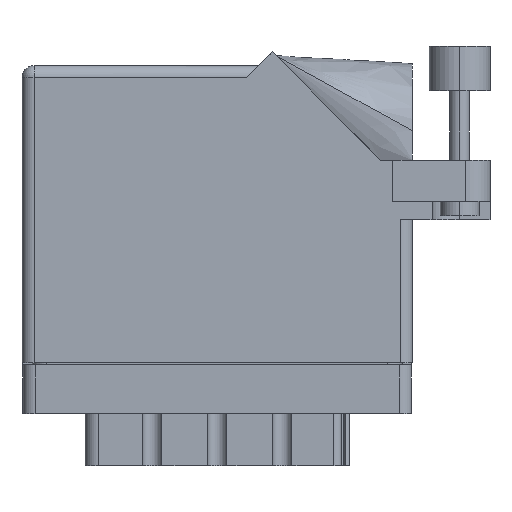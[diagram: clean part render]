
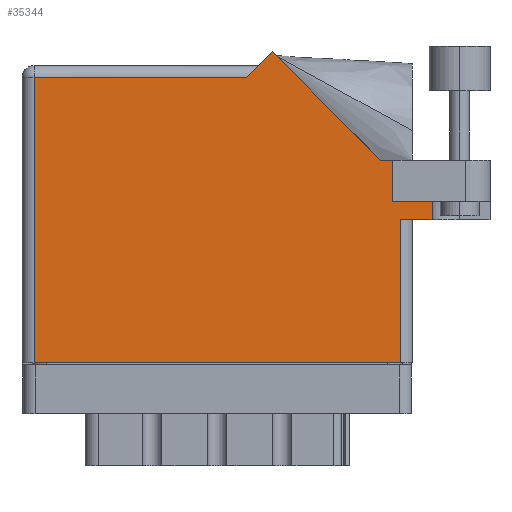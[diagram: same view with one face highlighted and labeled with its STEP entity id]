
A CAD part, front view. The second image highlights one B-rep face of the part: STEP entity #35344.
In plain terms, the highlighted face is planar.
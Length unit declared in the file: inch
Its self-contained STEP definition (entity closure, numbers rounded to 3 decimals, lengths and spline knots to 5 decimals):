
#977 = VERTEX_POINT ( 'NONE', #35370 ) ;
#1041 = CARTESIAN_POINT ( 'NONE',  ( 1.948, 0.737, 0. ) ) ;
#1799 = DIRECTION ( 'NONE',  ( 1., 0., 0. ) ) ;
#2195 = VECTOR ( 'NONE', #29705, 39.37008 ) ;
#2524 = CARTESIAN_POINT ( 'NONE',  ( 1.91, 0.831, 0. ) ) ;
#3030 = LINE ( 'NONE', #2524, #31104 ) ;
#3274 = VECTOR ( 'NONE', #40056, 39.37008 ) ;
#3302 = DIRECTION ( 'NONE',  ( 0., 0., -1. ) ) ;
#3703 = ORIENTED_EDGE ( 'NONE', *, *, #16335, .F. ) ;
#4080 = DIRECTION ( 'NONE',  ( -0.707, -0.707, 0. ) ) ;
#4946 = EDGE_CURVE ( 'NONE', #19174, #19849, #27779, .T. ) ;
#5634 = CARTESIAN_POINT ( 'NONE',  ( 1.84442, 1.044, 0. ) ) ;
#6701 = EDGE_CURVE ( 'NONE', #10170, #16494, #29284, .T. ) ;
#7838 = CARTESIAN_POINT ( 'NONE',  ( 2.01, 0.737, 0. ) ) ;
#8019 = VECTOR ( 'NONE', #28084, 39.37008 ) ;
#8037 = CARTESIAN_POINT ( 'NONE',  ( 1.84442, 1.044, 0. ) ) ;
#10122 = EDGE_CURVE ( 'NONE', #19849, #34673, #13090, .T. ) ;
#10170 = VERTEX_POINT ( 'NONE', #34140 ) ;
#11305 = DIRECTION ( 'NONE',  ( 0., -1., 0. ) ) ;
#11862 = CARTESIAN_POINT ( 'NONE',  ( 1.155, 1.468, 0. ) ) ;
#12029 = LINE ( 'NONE', #41518, #32100 ) ;
#12584 = LINE ( 'NONE', #23384, #13114 ) ;
#12904 = CARTESIAN_POINT ( 'NONE',  ( 1.28771, 1.60071, 0. ) ) ;
#13090 = LINE ( 'NONE', #5634, #8019 ) ;
#13114 = VECTOR ( 'NONE', #11305, 39.37008 ) ;
#13465 = EDGE_CURVE ( 'NONE', #977, #10170, #34619, .T. ) ;
#14250 = VERTEX_POINT ( 'NONE', #11862 ) ;
#14362 = VECTOR ( 'NONE', #4080, 39.37008 ) ;
#14633 = CARTESIAN_POINT ( 'NONE',  ( 1.948, 0., 0. ) ) ;
#15467 = ORIENTED_EDGE ( 'NONE', *, *, #37734, .T. ) ;
#15616 = VECTOR ( 'NONE', #40370, 39.37008 ) ;
#15752 = CARTESIAN_POINT ( 'NONE',  ( 2.1115, 0.831, 0. ) ) ;
#16335 = EDGE_CURVE ( 'NONE', #34590, #29541, #12029, .T. ) ;
#16494 = VERTEX_POINT ( 'NONE', #14633 ) ;
#17437 = EDGE_CURVE ( 'NONE', #32057, #32984, #25446, .T. ) ;
#17979 = CARTESIAN_POINT ( 'NONE',  ( 0., 1.468, 0. ) ) ;
#18394 = EDGE_CURVE ( 'NONE', #34673, #14250, #27894, .T. ) ;
#19174 = VERTEX_POINT ( 'NONE', #39757 ) ;
#19693 = CARTESIAN_POINT ( 'NONE',  ( 0., 1.53, 0. ) ) ;
#19698 = EDGE_LOOP ( 'NONE', ( #29198, #15467, #26949, #22063, #3703, #23926, #40928, #27675, #39932, #21300, #20784 ) ) ;
#19849 = VERTEX_POINT ( 'NONE', #8037 ) ;
#19925 = VECTOR ( 'NONE', #1799, 39.37008 ) ;
#20784 = ORIENTED_EDGE ( 'NONE', *, *, #13465, .T. ) ;
#20928 = DIRECTION ( 'NONE',  ( 1., 0., 0. ) ) ;
#21300 = ORIENTED_EDGE ( 'NONE', *, *, #29539, .T. ) ;
#22063 = ORIENTED_EDGE ( 'NONE', *, *, #23149, .F. ) ;
#22115 = CARTESIAN_POINT ( 'NONE',  ( 1.91, 0.831, 0. ) ) ;
#22775 = VECTOR ( 'NONE', #20928, 39.37008 ) ;
#23149 = EDGE_CURVE ( 'NONE', #29541, #32984, #12584, .T. ) ;
#23384 = CARTESIAN_POINT ( 'NONE',  ( 2.1115, 1.16177, 0. ) ) ;
#23541 = EDGE_CURVE ( 'NONE', #34590, #19174, #3030, .T. ) ;
#23926 = ORIENTED_EDGE ( 'NONE', *, *, #23541, .T. ) ;
#24104 = LINE ( 'NONE', #17979, #15616 ) ;
#25446 = LINE ( 'NONE', #7838, #19925 ) ;
#26949 = ORIENTED_EDGE ( 'NONE', *, *, #17437, .T. ) ;
#27675 = ORIENTED_EDGE ( 'NONE', *, *, #10122, .T. ) ;
#27779 = LINE ( 'NONE', #39233, #2195 ) ;
#27894 = LINE ( 'NONE', #39392, #14362 ) ;
#28084 = DIRECTION ( 'NONE',  ( -0.707, 0.707, 0. ) ) ;
#28973 = AXIS2_PLACEMENT_3D ( 'NONE', #19693, #3302, #32335 ) ;
#29198 = ORIENTED_EDGE ( 'NONE', *, *, #6701, .T. ) ;
#29284 = LINE ( 'NONE', #40127, #22775 ) ;
#29539 = EDGE_CURVE ( 'NONE', #14250, #977, #24104, .T. ) ;
#29541 = VERTEX_POINT ( 'NONE', #15752 ) ;
#29705 = DIRECTION ( 'NONE',  ( -1., 0., 0. ) ) ;
#30269 = CARTESIAN_POINT ( 'NONE',  ( 1.948, 0.737, 0. ) ) ;
#31104 = VECTOR ( 'NONE', #38386, 39.37008 ) ;
#31481 = CARTESIAN_POINT ( 'NONE',  ( 0.062, 0., 0. ) ) ;
#32057 = VERTEX_POINT ( 'NONE', #1041 ) ;
#32100 = VECTOR ( 'NONE', #38863, 39.37008 ) ;
#32335 = DIRECTION ( 'NONE',  ( -1., 0., 0. ) ) ;
#32984 = VERTEX_POINT ( 'NONE', #35993 ) ;
#34119 = VECTOR ( 'NONE', #38738, 39.37008 ) ;
#34140 = CARTESIAN_POINT ( 'NONE',  ( 0.062, 0., 0. ) ) ;
#34590 = VERTEX_POINT ( 'NONE', #22115 ) ;
#34619 = LINE ( 'NONE', #31481, #34119 ) ;
#34673 = VERTEX_POINT ( 'NONE', #12904 ) ;
#35344 = ADVANCED_FACE ( 'NONE', ( #36517 ), #35405, .F. ) ;
#35370 = CARTESIAN_POINT ( 'NONE',  ( 0.062, 1.468, 0. ) ) ;
#35405 = PLANE ( 'NONE',  #28973 ) ;
#35993 = CARTESIAN_POINT ( 'NONE',  ( 2.1115, 0.737, 0. ) ) ;
#36517 = FACE_OUTER_BOUND ( 'NONE', #19698, .T. ) ;
#37368 = LINE ( 'NONE', #30269, #3274 ) ;
#37734 = EDGE_CURVE ( 'NONE', #16494, #32057, #37368, .T. ) ;
#38386 = DIRECTION ( 'NONE',  ( 0., 1., 0. ) ) ;
#38738 = DIRECTION ( 'NONE',  ( 0., -1., 0. ) ) ;
#38863 = DIRECTION ( 'NONE',  ( 1., 0., 0. ) ) ;
#39233 = CARTESIAN_POINT ( 'NONE',  ( 2.41, 1.044, 0. ) ) ;
#39392 = CARTESIAN_POINT ( 'NONE',  ( 1.217, 1.53, 0. ) ) ;
#39757 = CARTESIAN_POINT ( 'NONE',  ( 1.91, 1.044, 0. ) ) ;
#39932 = ORIENTED_EDGE ( 'NONE', *, *, #18394, .T. ) ;
#40056 = DIRECTION ( 'NONE',  ( 0., 1., 0. ) ) ;
#40127 = CARTESIAN_POINT ( 'NONE',  ( 0., 0., 0. ) ) ;
#40370 = DIRECTION ( 'NONE',  ( -1., 0., 0. ) ) ;
#40928 = ORIENTED_EDGE ( 'NONE', *, *, #4946, .T. ) ;
#41518 = CARTESIAN_POINT ( 'NONE',  ( 1.91, 0.831, 0. ) ) ;
